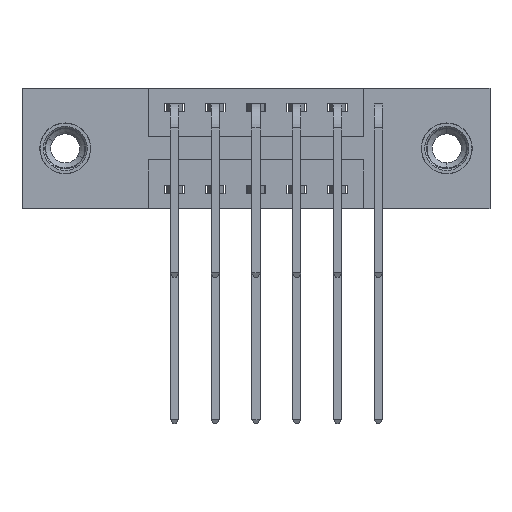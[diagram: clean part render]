
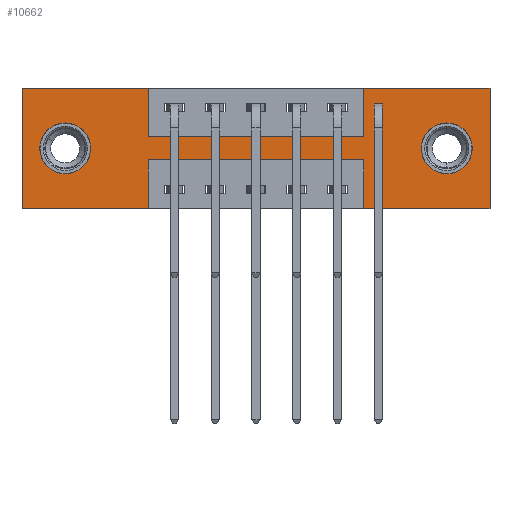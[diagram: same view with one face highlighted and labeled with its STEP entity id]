
A CAD part, front view. The second image highlights one B-rep face of the part: STEP entity #10662.
In plain terms, the highlighted planar face has unit normal (0, -1, 0).
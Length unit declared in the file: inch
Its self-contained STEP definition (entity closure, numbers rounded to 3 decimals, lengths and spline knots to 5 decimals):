
#5 = CARTESIAN_POINT ( 'NONE',  ( 1.0475, 0., -0.37 ) ) ;
#147 = EDGE_CURVE ( 'NONE', #5783, #5088, #10046, .T. ) ;
#159 = EDGE_CURVE ( 'NONE', #758, #5783, #9233, .T. ) ;
#308 = CARTESIAN_POINT ( 'NONE',  ( 0.1325, 0., -0.107 ) ) ;
#422 = VECTOR ( 'NONE', #3116, 39.37008 ) ;
#487 = CARTESIAN_POINT ( 'NONE',  ( 1.3025, 0., -0.185 ) ) ;
#758 = VERTEX_POINT ( 'NONE', #9546 ) ;
#855 = EDGE_CURVE ( 'NONE', #10192, #3599, #1938, .T. ) ;
#860 = EDGE_CURVE ( 'NONE', #8780, #9866, #8920, .T. ) ;
#1025 = CARTESIAN_POINT ( 'NONE',  ( 1.3025, 0., -0.185 ) ) ;
#1137 = VERTEX_POINT ( 'NONE', #3490 ) ;
#1341 = CARTESIAN_POINT ( 'NONE',  ( 0.1325, 0., -0.263 ) ) ;
#1374 = DIRECTION ( 'NONE',  ( -1., 0., 0. ) ) ;
#1375 = EDGE_CURVE ( 'NONE', #4931, #1542, #3390, .T. ) ;
#1384 = CARTESIAN_POINT ( 'NONE',  ( 1.0475, 0., -0.22 ) ) ;
#1477 = ORIENTED_EDGE ( 'NONE', *, *, #2581, .F. ) ;
#1499 = CARTESIAN_POINT ( 'NONE',  ( 0., 0., 0. ) ) ;
#1542 = VERTEX_POINT ( 'NONE', #9178 ) ;
#1544 = DIRECTION ( 'NONE',  ( 0., -1., 0. ) ) ;
#1838 = DIRECTION ( 'NONE',  ( 0., 0., 1. ) ) ;
#1862 = ORIENTED_EDGE ( 'NONE', *, *, #6402, .F. ) ;
#1910 = ORIENTED_EDGE ( 'NONE', *, *, #10952, .F. ) ;
#1938 = LINE ( 'NONE', #2862, #8146 ) ;
#1942 = CARTESIAN_POINT ( 'NONE',  ( 1.0475, 0., -0.15 ) ) ;
#2056 = CARTESIAN_POINT ( 'NONE',  ( 0.3875, 0., -0.37 ) ) ;
#2173 = DIRECTION ( 'NONE',  ( 0., 0., 1. ) ) ;
#2293 = LINE ( 'NONE', #8705, #10416 ) ;
#2343 = DIRECTION ( 'NONE',  ( 0., 0., -1. ) ) ;
#2403 = FACE_OUTER_BOUND ( 'NONE', #3716, .T. ) ;
#2420 = EDGE_CURVE ( 'NONE', #4578, #8840, #9786, .T. ) ;
#2581 = EDGE_CURVE ( 'NONE', #6486, #8780, #8489, .T. ) ;
#2767 = ORIENTED_EDGE ( 'NONE', *, *, #147, .F. ) ;
#2801 = VECTOR ( 'NONE', #10270, 39.37008 ) ;
#2856 = LINE ( 'NONE', #7313, #7031 ) ;
#2862 = CARTESIAN_POINT ( 'NONE',  ( 0.3875, 0., -0.37 ) ) ;
#3116 = DIRECTION ( 'NONE',  ( -1., 0., 0. ) ) ;
#3357 = ORIENTED_EDGE ( 'NONE', *, *, #1375, .T. ) ;
#3390 = CIRCLE ( 'NONE', #8522, 0.078 ) ;
#3490 = CARTESIAN_POINT ( 'NONE',  ( 0., 0., -0.37 ) ) ;
#3517 = EDGE_CURVE ( 'NONE', #8840, #4578, #9273, .T. ) ;
#3599 = VERTEX_POINT ( 'NONE', #2056 ) ;
#3716 = EDGE_LOOP ( 'NONE', ( #9764, #4038, #2767, #6710, #1910, #1862, #3755, #8488, #8113, #1477, #4682, #8615 ) ) ;
#3724 = DIRECTION ( 'NONE',  ( -1., 0., 0. ) ) ;
#3755 = ORIENTED_EDGE ( 'NONE', *, *, #8876, .F. ) ;
#3966 = DIRECTION ( 'NONE',  ( 0., 1., 0. ) ) ;
#4013 = VERTEX_POINT ( 'NONE', #10963 ) ;
#4038 = ORIENTED_EDGE ( 'NONE', *, *, #9227, .F. ) ;
#4115 = LINE ( 'NONE', #4743, #10238 ) ;
#4358 = AXIS2_PLACEMENT_3D ( 'NONE', #7985, #8087, #1838 ) ;
#4382 = CARTESIAN_POINT ( 'NONE',  ( 0.3875, 0., -0.15 ) ) ;
#4516 = DIRECTION ( 'NONE',  ( 0., 1., 0. ) ) ;
#4578 = VERTEX_POINT ( 'NONE', #1341 ) ;
#4579 = LINE ( 'NONE', #7153, #7920 ) ;
#4682 = ORIENTED_EDGE ( 'NONE', *, *, #7548, .F. ) ;
#4723 = AXIS2_PLACEMENT_3D ( 'NONE', #9378, #1544, #2343 ) ;
#4743 = CARTESIAN_POINT ( 'NONE',  ( 0., 0., -0.37 ) ) ;
#4931 = VERTEX_POINT ( 'NONE', #5390 ) ;
#5038 = VERTEX_POINT ( 'NONE', #10990 ) ;
#5088 = VERTEX_POINT ( 'NONE', #1384 ) ;
#5204 = DIRECTION ( 'NONE',  ( 1., 0., 0. ) ) ;
#5314 = VECTOR ( 'NONE', #8557, 39.37008 ) ;
#5390 = CARTESIAN_POINT ( 'NONE',  ( 1.3025, 0., -0.263 ) ) ;
#5391 = CARTESIAN_POINT ( 'NONE',  ( 0.1325, 0., -0.185 ) ) ;
#5783 = VERTEX_POINT ( 'NONE', #5 ) ;
#5960 = CARTESIAN_POINT ( 'NONE',  ( 0.3875, 0., -0.22 ) ) ;
#6327 = DIRECTION ( 'NONE',  ( 0., 0., -1. ) ) ;
#6334 = CARTESIAN_POINT ( 'NONE',  ( 0.3875, 0., 0. ) ) ;
#6392 = DIRECTION ( 'NONE',  ( 0., 0., -1. ) ) ;
#6402 = EDGE_CURVE ( 'NONE', #5038, #4013, #2293, .T. ) ;
#6486 = VERTEX_POINT ( 'NONE', #9448 ) ;
#6512 = EDGE_LOOP ( 'NONE', ( #8482, #3357 ) ) ;
#6622 = CIRCLE ( 'NONE', #7742, 0.078 ) ;
#6691 = EDGE_CURVE ( 'NONE', #3599, #1137, #4115, .T. ) ;
#6710 = ORIENTED_EDGE ( 'NONE', *, *, #159, .F. ) ;
#7031 = VECTOR ( 'NONE', #6327, 39.37008 ) ;
#7153 = CARTESIAN_POINT ( 'NONE',  ( 0.3875, 0., -0.22 ) ) ;
#7313 = CARTESIAN_POINT ( 'NONE',  ( 1.435, 0., 0. ) ) ;
#7446 = DIRECTION ( 'NONE',  ( 0., 0., -1. ) ) ;
#7463 = CARTESIAN_POINT ( 'NONE',  ( 1.0475, 0., -0.37 ) ) ;
#7548 = EDGE_CURVE ( 'NONE', #1137, #6486, #9607, .T. ) ;
#7569 = LINE ( 'NONE', #9401, #2801 ) ;
#7742 = AXIS2_PLACEMENT_3D ( 'NONE', #487, #3966, #7446 ) ;
#7914 = DIRECTION ( 'NONE',  ( 1., 0., 0. ) ) ;
#7920 = VECTOR ( 'NONE', #3724, 39.37008 ) ;
#7951 = VECTOR ( 'NONE', #2173, 39.37008 ) ;
#7985 = CARTESIAN_POINT ( 'NONE',  ( 0.1325, 0., -0.185 ) ) ;
#8076 = DIRECTION ( 'NONE',  ( 0., 0., -1. ) ) ;
#8087 = DIRECTION ( 'NONE',  ( 0., 1., 0. ) ) ;
#8113 = ORIENTED_EDGE ( 'NONE', *, *, #860, .F. ) ;
#8146 = VECTOR ( 'NONE', #8076, 39.37008 ) ;
#8482 = ORIENTED_EDGE ( 'NONE', *, *, #10110, .T. ) ;
#8488 = ORIENTED_EDGE ( 'NONE', *, *, #8529, .F. ) ;
#8489 = LINE ( 'NONE', #1499, #10547 ) ;
#8522 = AXIS2_PLACEMENT_3D ( 'NONE', #1025, #4516, #9807 ) ;
#8529 = EDGE_CURVE ( 'NONE', #9866, #9300, #7569, .T. ) ;
#8557 = DIRECTION ( 'NONE',  ( 0., 0., 1. ) ) ;
#8615 = ORIENTED_EDGE ( 'NONE', *, *, #6691, .F. ) ;
#8705 = CARTESIAN_POINT ( 'NONE',  ( 0., 0., 0. ) ) ;
#8780 = VERTEX_POINT ( 'NONE', #10770 ) ;
#8840 = VERTEX_POINT ( 'NONE', #308 ) ;
#8876 = EDGE_CURVE ( 'NONE', #9300, #5038, #10020, .T. ) ;
#8884 = DIRECTION ( 'NONE',  ( 0., 1., 0. ) ) ;
#8920 = LINE ( 'NONE', #6334, #11060 ) ;
#9003 = VECTOR ( 'NONE', #9121, 39.37008 ) ;
#9121 = DIRECTION ( 'NONE',  ( 0., 0., 1. ) ) ;
#9156 = EDGE_LOOP ( 'NONE', ( #9622, #11254 ) ) ;
#9178 = CARTESIAN_POINT ( 'NONE',  ( 1.3025, 0., -0.107 ) ) ;
#9227 = EDGE_CURVE ( 'NONE', #5088, #10192, #4579, .T. ) ;
#9233 = LINE ( 'NONE', #9289, #422 ) ;
#9273 = CIRCLE ( 'NONE', #4358, 0.078 ) ;
#9289 = CARTESIAN_POINT ( 'NONE',  ( 0., 0., -0.37 ) ) ;
#9300 = VERTEX_POINT ( 'NONE', #1942 ) ;
#9378 = CARTESIAN_POINT ( 'NONE',  ( 0., 0., -0.37 ) ) ;
#9401 = CARTESIAN_POINT ( 'NONE',  ( 0.3875, 0., -0.15 ) ) ;
#9440 = PLANE ( 'NONE',  #4723 ) ;
#9442 = AXIS2_PLACEMENT_3D ( 'NONE', #5391, #8884, #9783 ) ;
#9448 = CARTESIAN_POINT ( 'NONE',  ( 0., 0., 0. ) ) ;
#9546 = CARTESIAN_POINT ( 'NONE',  ( 1.435, 0., -0.37 ) ) ;
#9607 = LINE ( 'NONE', #10264, #5314 ) ;
#9622 = ORIENTED_EDGE ( 'NONE', *, *, #3517, .T. ) ;
#9764 = ORIENTED_EDGE ( 'NONE', *, *, #855, .F. ) ;
#9783 = DIRECTION ( 'NONE',  ( 0., 0., 1. ) ) ;
#9786 = CIRCLE ( 'NONE', #9442, 0.078 ) ;
#9807 = DIRECTION ( 'NONE',  ( 0., 0., -1. ) ) ;
#9866 = VERTEX_POINT ( 'NONE', #4382 ) ;
#9962 = CARTESIAN_POINT ( 'NONE',  ( 1.0475, 0., 0. ) ) ;
#10020 = LINE ( 'NONE', #9962, #7951 ) ;
#10046 = LINE ( 'NONE', #7463, #9003 ) ;
#10110 = EDGE_CURVE ( 'NONE', #1542, #4931, #6622, .T. ) ;
#10192 = VERTEX_POINT ( 'NONE', #5960 ) ;
#10238 = VECTOR ( 'NONE', #1374, 39.37008 ) ;
#10247 = FACE_BOUND ( 'NONE', #6512, .T. ) ;
#10264 = CARTESIAN_POINT ( 'NONE',  ( 0., 0., 0. ) ) ;
#10270 = DIRECTION ( 'NONE',  ( 1., 0., 0. ) ) ;
#10303 = FACE_BOUND ( 'NONE', #9156, .T. ) ;
#10416 = VECTOR ( 'NONE', #7914, 39.37008 ) ;
#10547 = VECTOR ( 'NONE', #5204, 39.37008 ) ;
#10662 = ADVANCED_FACE ( 'NONE', ( #10247, #10303, #2403 ), #9440, .T. ) ;
#10770 = CARTESIAN_POINT ( 'NONE',  ( 0.3875, 0., 0. ) ) ;
#10952 = EDGE_CURVE ( 'NONE', #4013, #758, #2856, .T. ) ;
#10963 = CARTESIAN_POINT ( 'NONE',  ( 1.435, 0., 0. ) ) ;
#10990 = CARTESIAN_POINT ( 'NONE',  ( 1.0475, 0., 0. ) ) ;
#11060 = VECTOR ( 'NONE', #6392, 39.37008 ) ;
#11254 = ORIENTED_EDGE ( 'NONE', *, *, #2420, .T. ) ;
